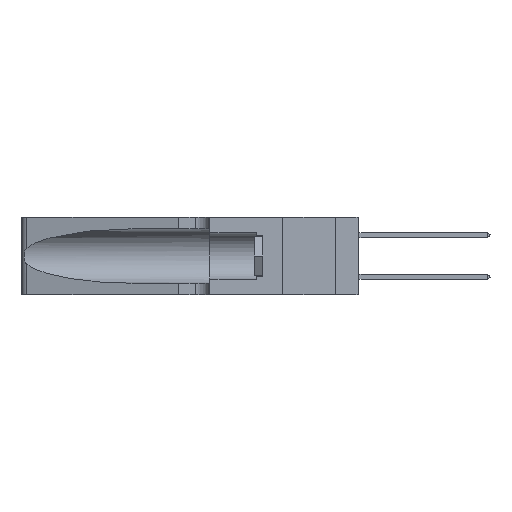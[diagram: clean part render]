
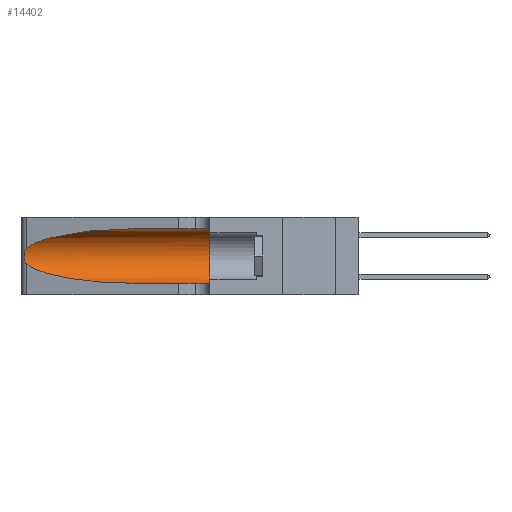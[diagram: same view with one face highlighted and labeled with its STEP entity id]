
A CAD part, left-side view. The second image highlights one B-rep face of the part: STEP entity #14402.
In plain terms, the highlighted cylindrical face has radius 3.308 mm (diameter 6.617 mm), a partial arc.
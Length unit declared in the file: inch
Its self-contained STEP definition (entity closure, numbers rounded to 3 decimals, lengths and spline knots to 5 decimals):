
#365 = AXIS2_PLACEMENT_3D ( 'NONE', #10086, #18845, #22913 ) ;
#534 = EDGE_LOOP ( 'NONE', ( #15434, #2292, #8097, #7068, #12032, #21640 ) ) ;
#1771 = CARTESIAN_POINT ( 'NONE',  ( 0.18966, 0.96281, 0.05475 ) ) ;
#1957 = CARTESIAN_POINT ( 'NONE',  ( 0.25787, 1.23484, 0.2124 ) ) ;
#2127 = CARTESIAN_POINT ( 'NONE',  ( 0.25789, 1.23486, 0.15765 ) ) ;
#2133 = VERTEX_POINT ( 'NONE', #8272 ) ;
#2292 = ORIENTED_EDGE ( 'NONE', *, *, #4616, .T. ) ;
#2431 = CARTESIAN_POINT ( 'NONE',  ( 0.25487, 1.22718, 0.22369 ) ) ;
#3322 = EDGE_CURVE ( 'NONE', #12689, #19724, #23559, .T. ) ;
#3444 = FACE_OUTER_BOUND ( 'NONE', #534, .T. ) ;
#3785 = CARTESIAN_POINT ( 'NONE',  ( 0.2373, 1.15595, 0.28018 ) ) ;
#4358 = CARTESIAN_POINT ( 'NONE',  ( 0.25856, 1.23593, 0.16098 ) ) ;
#4616 = EDGE_CURVE ( 'NONE', #2133, #5552, #22247, .T. ) ;
#4649 = VECTOR ( 'NONE', #10740, 39.37008 ) ;
#4842 = CARTESIAN_POINT ( 'NONE',  ( 0.1305, 1.61858, 0.185 ) ) ;
#4897 =( BOUNDED_CURVE ( )  B_SPLINE_CURVE ( 3, ( #15602, #26693, #1771, #17033 ),
 .UNSPECIFIED., .F., .F. ) 
 B_SPLINE_CURVE_WITH_KNOTS ( ( 4, 4 ),
 ( 3.44316, 4.71239 ),
 .UNSPECIFIED. ) 
 CURVE ( )  GEOMETRIC_REPRESENTATION_ITEM ( )  RATIONAL_B_SPLINE_CURVE ( ( 1., 0.87, 0.87, 1. ) ) 
 REPRESENTATION_ITEM ( '' )  );
#5552 = VERTEX_POINT ( 'NONE', #8719 ) ;
#5804 = CARTESIAN_POINT ( 'NONE',  ( 0.18966, 0.96281, 0.31525 ) ) ;
#6272 = CARTESIAN_POINT ( 'NONE',  ( 0.1305, 0.72297, 0.31525 ) ) ;
#6944 = DIRECTION ( 'NONE',  ( 0., 0., -1. ) ) ;
#7068 = ORIENTED_EDGE ( 'NONE', *, *, #7377, .T. ) ;
#7377 = EDGE_CURVE ( 'NONE', #13970, #19724, #23256, .T. ) ;
#8018 = CARTESIAN_POINT ( 'NONE',  ( 0.1305, 0.72297, 0.31525 ) ) ;
#8097 = ORIENTED_EDGE ( 'NONE', *, *, #17220, .T. ) ;
#8272 = CARTESIAN_POINT ( 'NONE',  ( 0.25487, 1.22718, 0.22369 ) ) ;
#8544 = CARTESIAN_POINT ( 'NONE',  ( 0.25639, 1.23184, 0.21858 ) ) ;
#8622 = CARTESIAN_POINT ( 'NONE',  ( 0.1305, 1.61858, 0.31525 ) ) ;
#8719 = CARTESIAN_POINT ( 'NONE',  ( 0.25487, 1.22718, 0.14631 ) ) ;
#9602 = CARTESIAN_POINT ( 'NONE',  ( 0.1305, 1.61858, 0.05475 ) ) ;
#10086 = CARTESIAN_POINT ( 'NONE',  ( 0.1305, 0.35, 0.185 ) ) ;
#10379 = CARTESIAN_POINT ( 'NONE',  ( 0.25555, 1.22994, 0.2215 ) ) ;
#10662 = CARTESIAN_POINT ( 'NONE',  ( 0.26075, 1.23896, 0.178 ) ) ;
#10740 = DIRECTION ( 'NONE',  ( 0., -1., 0. ) ) ;
#11781 = CARTESIAN_POINT ( 'NONE',  ( 0.1305, 0.35, 0.31525 ) ) ;
#12032 = ORIENTED_EDGE ( 'NONE', *, *, #3322, .F. ) ;
#12547 = CARTESIAN_POINT ( 'NONE',  ( 0.26018, 1.23835, 0.19895 ) ) ;
#12610 = CARTESIAN_POINT ( 'NONE',  ( 0.1305, 0.72297, 0.05475 ) ) ;
#12689 = VERTEX_POINT ( 'NONE', #11781 ) ;
#13970 = VERTEX_POINT ( 'NONE', #12610 ) ;
#14095 = VERTEX_POINT ( 'NONE', #6272 ) ;
#14402 = ADVANCED_FACE ( 'NONE', ( #3444 ), #18047, .F. ) ;
#14898 = CARTESIAN_POINT ( 'NONE',  ( 0.26075, 1.23896, 0.19203 ) ) ;
#14978 = VECTOR ( 'NONE', #22241, 39.37008 ) ;
#15434 = ORIENTED_EDGE ( 'NONE', *, *, #18200, .T. ) ;
#15602 = CARTESIAN_POINT ( 'NONE',  ( 0.25487, 1.22718, 0.14631 ) ) ;
#16186 = EDGE_CURVE ( 'NONE', #14095, #12689, #22621, .T. ) ;
#16337 = CARTESIAN_POINT ( 'NONE',  ( 0.25487, 1.22718, 0.22369 ) ) ;
#17033 = CARTESIAN_POINT ( 'NONE',  ( 0.1305, 0.72297, 0.05475 ) ) ;
#17220 = EDGE_CURVE ( 'NONE', #5552, #13970, #4897, .T. ) ;
#18047 = CYLINDRICAL_SURFACE ( 'NONE', #25699, 0.13025 ) ;
#18200 = EDGE_CURVE ( 'NONE', #14095, #2133, #27478, .T. ) ;
#18845 = DIRECTION ( 'NONE',  ( 0., 1., 0. ) ) ;
#19696 = DIRECTION ( 'NONE',  ( 0., -1., 0. ) ) ;
#19724 = VERTEX_POINT ( 'NONE', #26446 ) ;
#21640 = ORIENTED_EDGE ( 'NONE', *, *, #16186, .F. ) ;
#22241 = DIRECTION ( 'NONE',  ( 0., -1., 0. ) ) ;
#22247 = B_SPLINE_CURVE_WITH_KNOTS ( 'NONE', 3,
 ( #2431, #10379, #8544, #1957, #23396, #12547, #14898, #10662, #23219, #4358, #2127, #25432, #25339, #27368 ),
 .UNSPECIFIED., .F., .F.,
 ( 4, 2, 2, 2, 2, 2, 4 ),
 ( 0., 0.00027, 0.00053, 0.00107, 0.0016, 0.00187, 0.00214 ),
 .UNSPECIFIED. ) ;
#22621 = LINE ( 'NONE', #8622, #4649 ) ;
#22913 = DIRECTION ( 'NONE',  ( 0., 0., 1. ) ) ;
#23219 = CARTESIAN_POINT ( 'NONE',  ( 0.26017, 1.23833, 0.17102 ) ) ;
#23256 = LINE ( 'NONE', #9602, #14978 ) ;
#23396 = CARTESIAN_POINT ( 'NONE',  ( 0.25854, 1.2359, 0.20912 ) ) ;
#23559 = CIRCLE ( 'NONE', #365, 0.13025 ) ;
#25339 = CARTESIAN_POINT ( 'NONE',  ( 0.25555, 1.22993, 0.14849 ) ) ;
#25432 = CARTESIAN_POINT ( 'NONE',  ( 0.25639, 1.23186, 0.15144 ) ) ;
#25699 = AXIS2_PLACEMENT_3D ( 'NONE', #4842, #19696, #6944 ) ;
#26446 = CARTESIAN_POINT ( 'NONE',  ( 0.1305, 0.35, 0.05475 ) ) ;
#26693 = CARTESIAN_POINT ( 'NONE',  ( 0.2373, 1.15595, 0.08982 ) ) ;
#27368 = CARTESIAN_POINT ( 'NONE',  ( 0.25487, 1.22718, 0.14631 ) ) ;
#27478 =( BOUNDED_CURVE ( )  B_SPLINE_CURVE ( 3, ( #8018, #5804, #3785, #16337 ),
 .UNSPECIFIED., .F., .T. ) 
 B_SPLINE_CURVE_WITH_KNOTS ( ( 4, 4 ),
 ( 1.5708, 2.84003 ),
 .UNSPECIFIED. ) 
 CURVE ( )  GEOMETRIC_REPRESENTATION_ITEM ( )  RATIONAL_B_SPLINE_CURVE ( ( 1., 0.87, 0.87, 1. ) ) 
 REPRESENTATION_ITEM ( '' )  );
